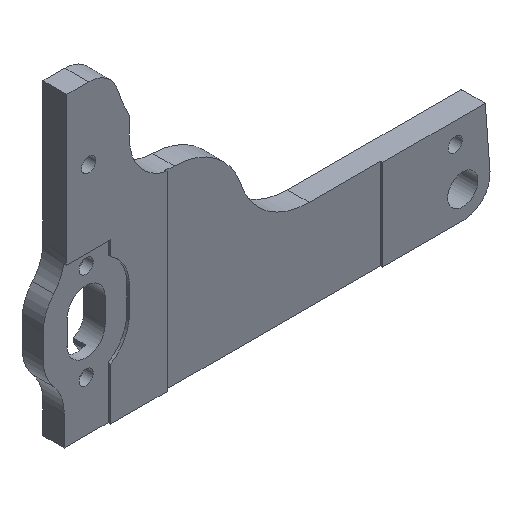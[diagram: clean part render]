
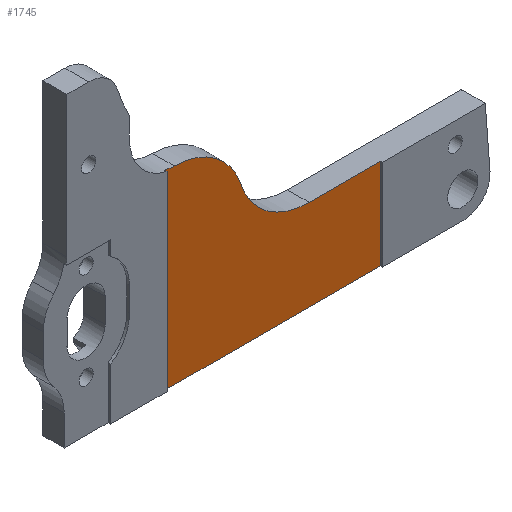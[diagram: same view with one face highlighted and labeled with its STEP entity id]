
A CAD part, isometric view. The second image highlights one B-rep face of the part: STEP entity #1745.
In plain terms, the highlighted planar face has unit normal (0, -1, 0).
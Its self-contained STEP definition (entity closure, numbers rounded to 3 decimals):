
#38 = VERTEX_POINT ( 'NONE', #489 ) ;
#40 = EDGE_CURVE ( 'NONE', #1203, #316, #638, .T. ) ;
#57 = DIRECTION ( 'NONE',  ( 0., 0., 1. ) ) ;
#62 = CARTESIAN_POINT ( 'NONE',  ( 51.219, 0.457, -45.387 ) ) ;
#142 = CARTESIAN_POINT ( 'NONE',  ( 21.006, 0.457, -24.424 ) ) ;
#169 = CARTESIAN_POINT ( 'NONE',  ( 23.132, 0.457, -14.653 ) ) ;
#179 = DIRECTION ( 'NONE',  ( 1., 0., 0. ) ) ;
#188 = AXIS2_PLACEMENT_3D ( 'NONE', #348, #311, #382 ) ;
#263 = EDGE_CURVE ( 'NONE', #1826, #1451, #1201, .T. ) ;
#311 = DIRECTION ( 'NONE',  ( 0., 1., 0. ) ) ;
#316 = VERTEX_POINT ( 'NONE', #442 ) ;
#318 = DIRECTION ( 'NONE',  ( 0., 0., 1. ) ) ;
#331 = VECTOR ( 'NONE', #179, 1000. ) ;
#348 = CARTESIAN_POINT ( 'NONE',  ( 51.219, 0.457, -30.387 ) ) ;
#359 = DIRECTION ( 'NONE',  ( 0., 0., 1. ) ) ;
#380 = AXIS2_PLACEMENT_3D ( 'NONE', #626, #1174, #57 ) ;
#382 = DIRECTION ( 'NONE',  ( 0., 0., 1. ) ) ;
#394 = DIRECTION ( 'NONE',  ( 0., 1., 0. ) ) ;
#407 = CARTESIAN_POINT ( 'NONE',  ( 22.685, 0.457, -39.649 ) ) ;
#442 = CARTESIAN_POINT ( 'NONE',  ( 36.952, 0.457, -35.018 ) ) ;
#489 = CARTESIAN_POINT ( 'NONE',  ( 22.953, 0.457, -24.651 ) ) ;
#562 = CARTESIAN_POINT ( 'NONE',  ( 0., 0.457, -45.387 ) ) ;
#603 = CIRCLE ( 'NONE', #2145, 15. ) ;
#626 = CARTESIAN_POINT ( 'NONE',  ( 0., 0.457, 0. ) ) ;
#638 = CIRCLE ( 'NONE', #188, 15. ) ;
#688 = DIRECTION ( 'NONE',  ( 0., 0., 1. ) ) ;
#717 = EDGE_LOOP ( 'NONE', ( #838, #1556, #1163, #735, #1993, #1544, #2233 ) ) ;
#735 = ORIENTED_EDGE ( 'NONE', *, *, #263, .T. ) ;
#755 = EDGE_CURVE ( 'NONE', #38, #316, #603, .T. ) ;
#838 = ORIENTED_EDGE ( 'NONE', *, *, #755, .F. ) ;
#850 = DIRECTION ( 'NONE',  ( 0., 0., 1. ) ) ;
#909 = VECTOR ( 'NONE', #850, 1000. ) ;
#953 = CARTESIAN_POINT ( 'NONE',  ( 0., 0.457, -64.364 ) ) ;
#1163 = ORIENTED_EDGE ( 'NONE', *, *, #1930, .F. ) ;
#1174 = DIRECTION ( 'NONE',  ( 0., 1., 0. ) ) ;
#1201 = LINE ( 'NONE', #953, #1262 ) ;
#1203 = VERTEX_POINT ( 'NONE', #62 ) ;
#1262 = VECTOR ( 'NONE', #2130, 1000. ) ;
#1308 = LINE ( 'NONE', #562, #331 ) ;
#1441 = DIRECTION ( 'NONE',  ( 0., 1., 0. ) ) ;
#1451 = VERTEX_POINT ( 'NONE', #2111 ) ;
#1492 = EDGE_CURVE ( 'NONE', #38, #2005, #2007, .T. ) ;
#1544 = ORIENTED_EDGE ( 'NONE', *, *, #2102, .F. ) ;
#1556 = ORIENTED_EDGE ( 'NONE', *, *, #1492, .T. ) ;
#1735 = VECTOR ( 'NONE', #688, 1000. ) ;
#1745 = ADVANCED_FACE ( 'NONE', ( #2163 ), #2204, .F. ) ;
#1752 = CARTESIAN_POINT ( 'NONE',  ( 21.006, 0.457, 0. ) ) ;
#1826 = VERTEX_POINT ( 'NONE', #1887 ) ;
#1845 = LINE ( 'NONE', #1909, #909 ) ;
#1887 = CARTESIAN_POINT ( 'NONE',  ( 21.006, 0.457, -64.364 ) ) ;
#1898 = EDGE_CURVE ( 'NONE', #1451, #2198, #1845, .T. ) ;
#1903 = AXIS2_PLACEMENT_3D ( 'NONE', #169, #1441, #359 ) ;
#1909 = CARTESIAN_POINT ( 'NONE',  ( 66.167, 0.457, 0. ) ) ;
#1930 = EDGE_CURVE ( 'NONE', #1826, #2005, #2137, .T. ) ;
#1993 = ORIENTED_EDGE ( 'NONE', *, *, #1898, .T. ) ;
#2005 = VERTEX_POINT ( 'NONE', #142 ) ;
#2007 = CIRCLE ( 'NONE', #1903, 10. ) ;
#2102 = EDGE_CURVE ( 'NONE', #1203, #2198, #1308, .T. ) ;
#2111 = CARTESIAN_POINT ( 'NONE',  ( 66.167, 0.457, -64.364 ) ) ;
#2130 = DIRECTION ( 'NONE',  ( 1., 0., 0. ) ) ;
#2137 = LINE ( 'NONE', #1752, #1735 ) ;
#2145 = AXIS2_PLACEMENT_3D ( 'NONE', #407, #394, #318 ) ;
#2160 = CARTESIAN_POINT ( 'NONE',  ( 66.167, 0.457, -45.387 ) ) ;
#2163 = FACE_OUTER_BOUND ( 'NONE', #717, .T. ) ;
#2198 = VERTEX_POINT ( 'NONE', #2160 ) ;
#2204 = PLANE ( 'NONE',  #380 ) ;
#2233 = ORIENTED_EDGE ( 'NONE', *, *, #40, .T. ) ;
